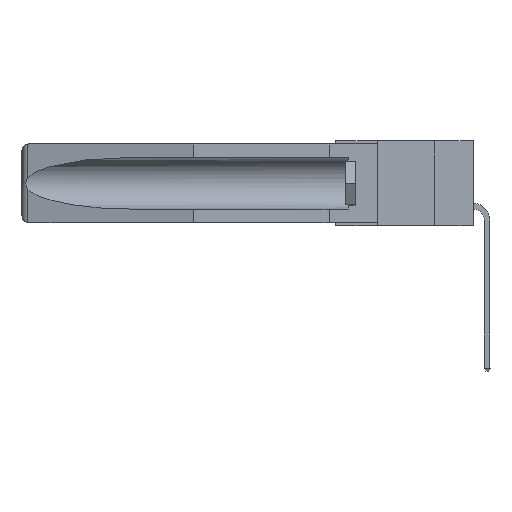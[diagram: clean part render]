
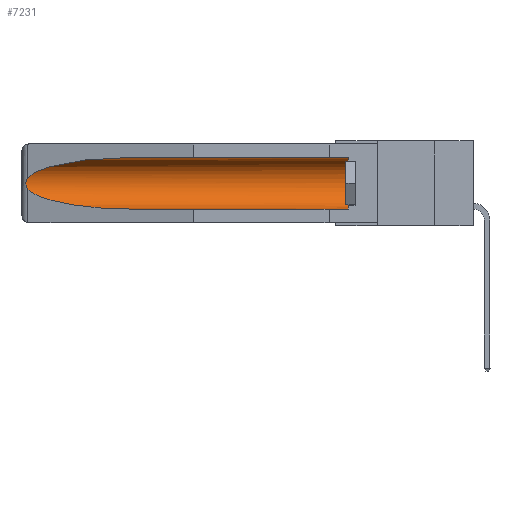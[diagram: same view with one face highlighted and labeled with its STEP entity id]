
A CAD part, left-side view. The second image highlights one B-rep face of the part: STEP entity #7231.
In plain terms, the highlighted cylindrical face has radius 2.857 mm (diameter 5.715 mm), a partial arc.
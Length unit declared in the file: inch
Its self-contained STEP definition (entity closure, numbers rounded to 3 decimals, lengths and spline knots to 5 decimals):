
#1598 = VERTEX_POINT ( 'NONE', #24930 ) ;
#1824 = CARTESIAN_POINT ( 'NONE',  ( 0.155, 1.07973, -0.059 ) ) ;
#2296 = B_SPLINE_CURVE_WITH_KNOTS ( 'NONE', 3,
 ( #6367, #20310, #8382, #20064, #22272, #14320, #20651, #24801, #10474, #4600 ),
 .UNSPECIFIED., .F., .F.,
 ( 4, 2, 2, 2, 4 ),
 ( 0., 0.00029, 0.00058, 0.00087, 0.00117 ),
 .UNSPECIFIED. ) ;
#2992 = VERTEX_POINT ( 'NONE', #14097 ) ;
#3568 = CARTESIAN_POINT ( 'NONE',  ( 0.25451, 1.48313, -0.09465 ) ) ;
#4341 = DIRECTION ( 'NONE',  ( 0., 0., 1. ) ) ;
#4600 = CARTESIAN_POINT ( 'NONE',  ( 0.26537, 1.52718, -0.19328 ) ) ;
#4603 = EDGE_CURVE ( 'NONE', #1598, #17551, #6625, .T. ) ;
#4958 = ORIENTED_EDGE ( 'NONE', *, *, #4603, .T. ) ;
#5333 =( BOUNDED_CURVE ( )  B_SPLINE_CURVE ( 3, ( #25693, #19792, #3568, #11533 ),
 .UNSPECIFIED., .F., .F. ) 
 B_SPLINE_CURVE_WITH_KNOTS ( ( 4, 4 ),
 ( 4.71239, 6.08839 ),
 .UNSPECIFIED. ) 
 CURVE ( )  GEOMETRIC_REPRESENTATION_ITEM ( )  RATIONAL_B_SPLINE_CURVE ( ( 1., 0.848, 0.848, 1. ) ) 
 REPRESENTATION_ITEM ( '' )  );
#5641 = AXIS2_PLACEMENT_3D ( 'NONE', #20530, #14796, #14709 ) ;
#5894 = VECTOR ( 'NONE', #19105, 39.37008 ) ;
#6367 = CARTESIAN_POINT ( 'NONE',  ( 0.26537, 1.52718, -0.14972 ) ) ;
#6538 = CARTESIAN_POINT ( 'NONE',  ( 0.21114, 1.30732, -0.284 ) ) ;
#6625 = CIRCLE ( 'NONE', #5641, 0.1125 ) ;
#7149 = CARTESIAN_POINT ( 'NONE',  ( 0.155, -0.30754, -0.059 ) ) ;
#7231 = ADVANCED_FACE ( 'NONE', ( #22129 ), #8985, .F. ) ;
#7674 = ORIENTED_EDGE ( 'NONE', *, *, #16490, .T. ) ;
#8382 = CARTESIAN_POINT ( 'NONE',  ( 0.26654, 1.53092, -0.15636 ) ) ;
#8985 = CYLINDRICAL_SURFACE ( 'NONE', #21230, 0.1125 ) ;
#9326 = LINE ( 'NONE', #7149, #5894 ) ;
#10474 = CARTESIAN_POINT ( 'NONE',  ( 0.26597, 1.5296, -0.19026 ) ) ;
#10592 = EDGE_CURVE ( 'NONE', #1598, #19989, #15551, .T. ) ;
#11192 = VERTEX_POINT ( 'NONE', #25881 ) ;
#11533 = CARTESIAN_POINT ( 'NONE',  ( 0.26537, 1.52718, -0.14972 ) ) ;
#12220 = DIRECTION ( 'NONE',  ( 0., 1., 0. ) ) ;
#12923 = EDGE_LOOP ( 'NONE', ( #18446, #23311, #15944, #21853, #4958, #7674 ) ) ;
#14097 = CARTESIAN_POINT ( 'NONE',  ( 0.26537, 1.52718, -0.14972 ) ) ;
#14320 = CARTESIAN_POINT ( 'NONE',  ( 0.2675, 1.53308, -0.17534 ) ) ;
#14709 = DIRECTION ( 'NONE',  ( 0., 0., 1. ) ) ;
#14757 = CARTESIAN_POINT ( 'NONE',  ( 0.25451, 1.48313, -0.24835 ) ) ;
#14796 = DIRECTION ( 'NONE',  ( 0., -1., 0. ) ) ;
#15076 = EDGE_CURVE ( 'NONE', #2992, #11192, #2296, .T. ) ;
#15551 = LINE ( 'NONE', #24032, #24290 ) ;
#15944 = ORIENTED_EDGE ( 'NONE', *, *, #22042, .T. ) ;
#16327 = DIRECTION ( 'NONE',  ( 0., 1., 0. ) ) ;
#16490 = EDGE_CURVE ( 'NONE', #17551, #16580, #9326, .T. ) ;
#16580 = VERTEX_POINT ( 'NONE', #1824 ) ;
#16672 = EDGE_CURVE ( 'NONE', #16580, #2992, #5333, .T. ) ;
#17551 = VERTEX_POINT ( 'NONE', #18020 ) ;
#18020 = CARTESIAN_POINT ( 'NONE',  ( 0.155, 0.126, -0.059 ) ) ;
#18303 = CARTESIAN_POINT ( 'NONE',  ( 0.155, 1.07973, -0.284 ) ) ;
#18446 = ORIENTED_EDGE ( 'NONE', *, *, #16672, .T. ) ;
#18933 =( BOUNDED_CURVE ( )  B_SPLINE_CURVE ( 3, ( #24474, #14757, #6538, #18303 ),
 .UNSPECIFIED., .F., .T. ) 
 B_SPLINE_CURVE_WITH_KNOTS ( ( 4, 4 ),
 ( 0.1948, 1.5708 ),
 .UNSPECIFIED. ) 
 CURVE ( )  GEOMETRIC_REPRESENTATION_ITEM ( )  RATIONAL_B_SPLINE_CURVE ( ( 1., 0.848, 0.848, 1. ) ) 
 REPRESENTATION_ITEM ( '' )  );
#19105 = DIRECTION ( 'NONE',  ( 0., 1., 0. ) ) ;
#19792 = CARTESIAN_POINT ( 'NONE',  ( 0.21114, 1.30732, -0.059 ) ) ;
#19989 = VERTEX_POINT ( 'NONE', #21798 ) ;
#20064 = CARTESIAN_POINT ( 'NONE',  ( 0.2673, 1.5327, -0.16383 ) ) ;
#20310 = CARTESIAN_POINT ( 'NONE',  ( 0.26597, 1.52961, -0.15275 ) ) ;
#20530 = CARTESIAN_POINT ( 'NONE',  ( 0.155, 0.126, -0.1715 ) ) ;
#20651 = CARTESIAN_POINT ( 'NONE',  ( 0.2673, 1.53269, -0.17917 ) ) ;
#21230 = AXIS2_PLACEMENT_3D ( 'NONE', #24044, #16327, #4341 ) ;
#21798 = CARTESIAN_POINT ( 'NONE',  ( 0.155, 1.07973, -0.284 ) ) ;
#21853 = ORIENTED_EDGE ( 'NONE', *, *, #10592, .F. ) ;
#22042 = EDGE_CURVE ( 'NONE', #11192, #19989, #18933, .T. ) ;
#22129 = FACE_OUTER_BOUND ( 'NONE', #12923, .T. ) ;
#22272 = CARTESIAN_POINT ( 'NONE',  ( 0.2675, 1.53308, -0.16763 ) ) ;
#23311 = ORIENTED_EDGE ( 'NONE', *, *, #15076, .T. ) ;
#24032 = CARTESIAN_POINT ( 'NONE',  ( 0.155, -0.30754, -0.284 ) ) ;
#24044 = CARTESIAN_POINT ( 'NONE',  ( 0.155, -0.30754, -0.1715 ) ) ;
#24290 = VECTOR ( 'NONE', #12220, 39.37008 ) ;
#24474 = CARTESIAN_POINT ( 'NONE',  ( 0.26537, 1.52718, -0.19328 ) ) ;
#24801 = CARTESIAN_POINT ( 'NONE',  ( 0.26655, 1.53094, -0.18657 ) ) ;
#24930 = CARTESIAN_POINT ( 'NONE',  ( 0.155, 0.126, -0.284 ) ) ;
#25693 = CARTESIAN_POINT ( 'NONE',  ( 0.155, 1.07973, -0.059 ) ) ;
#25881 = CARTESIAN_POINT ( 'NONE',  ( 0.26537, 1.52718, -0.19328 ) ) ;
